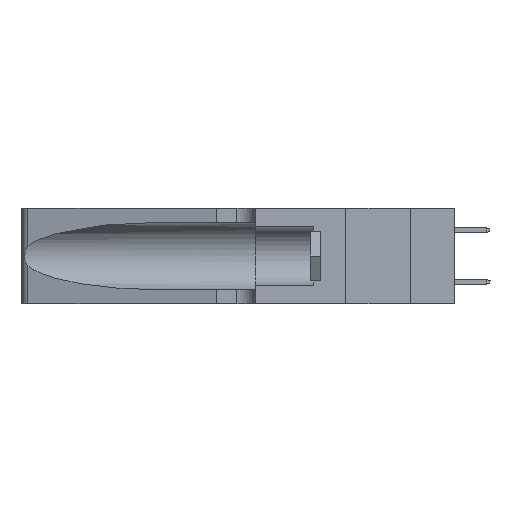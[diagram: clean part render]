
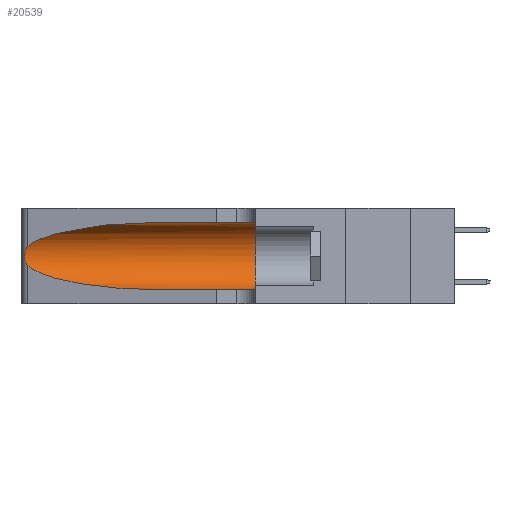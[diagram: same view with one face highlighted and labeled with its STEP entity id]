
A CAD part, left-side view. The second image highlights one B-rep face of the part: STEP entity #20539.
In plain terms, the highlighted cylindrical face has radius 3.308 mm (diameter 6.617 mm), a partial arc.
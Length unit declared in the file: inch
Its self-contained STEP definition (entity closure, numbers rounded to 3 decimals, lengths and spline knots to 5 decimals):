
#292 = CARTESIAN_POINT ( 'NONE',  ( 0.26075, 1.23896, 0.19203 ) ) ;
#440 = AXIS2_PLACEMENT_3D ( 'NONE', #18589, #21088, #26105 ) ;
#1150 = DIRECTION ( 'NONE',  ( 0., 0., -1. ) ) ;
#2036 = CARTESIAN_POINT ( 'NONE',  ( 0.1305, 0.72297, 0.05475 ) ) ;
#2188 = CARTESIAN_POINT ( 'NONE',  ( 0.1305, 1.61858, 0.31525 ) ) ;
#2453 = CARTESIAN_POINT ( 'NONE',  ( 0.25487, 1.22718, 0.22369 ) ) ;
#2631 = CARTESIAN_POINT ( 'NONE',  ( 0.25555, 1.22993, 0.14849 ) ) ;
#2704 = CARTESIAN_POINT ( 'NONE',  ( 0.1305, 0.35, 0.31525 ) ) ;
#2772 = CARTESIAN_POINT ( 'NONE',  ( 0.25787, 1.23484, 0.2124 ) ) ;
#3250 = VERTEX_POINT ( 'NONE', #12655 ) ;
#3545 = EDGE_CURVE ( 'NONE', #10088, #3250, #20313, .T. ) ;
#3621 = ORIENTED_EDGE ( 'NONE', *, *, #28173, .T. ) ;
#3912 = ORIENTED_EDGE ( 'NONE', *, *, #11905, .T. ) ;
#4317 = CARTESIAN_POINT ( 'NONE',  ( 0.25487, 1.22718, 0.22369 ) ) ;
#4674 = CARTESIAN_POINT ( 'NONE',  ( 0.2373, 1.15595, 0.08982 ) ) ;
#5006 = CARTESIAN_POINT ( 'NONE',  ( 0.25487, 1.22718, 0.14631 ) ) ;
#5049 = LINE ( 'NONE', #23955, #10799 ) ;
#5789 = FACE_OUTER_BOUND ( 'NONE', #12673, .T. ) ;
#5851 =( BOUNDED_CURVE ( )  B_SPLINE_CURVE ( 3, ( #9763, #19253, #19100, #2453 ),
 .UNSPECIFIED., .F., .F. ) 
 B_SPLINE_CURVE_WITH_KNOTS ( ( 4, 4 ),
 ( 1.5708, 2.84003 ),
 .UNSPECIFIED. ) 
 CURVE ( )  GEOMETRIC_REPRESENTATION_ITEM ( )  RATIONAL_B_SPLINE_CURVE ( ( 1., 0.87, 0.87, 1. ) ) 
 REPRESENTATION_ITEM ( '' )  );
#8058 =( BOUNDED_CURVE ( )  B_SPLINE_CURVE ( 3, ( #30767, #4674, #9676, #19167 ),
 .UNSPECIFIED., .F., .F. ) 
 B_SPLINE_CURVE_WITH_KNOTS ( ( 4, 4 ),
 ( 3.44316, 4.71239 ),
 .UNSPECIFIED. ) 
 CURVE ( )  GEOMETRIC_REPRESENTATION_ITEM ( )  RATIONAL_B_SPLINE_CURVE ( ( 1., 0.87, 0.87, 1. ) ) 
 REPRESENTATION_ITEM ( '' )  );
#8305 = DIRECTION ( 'NONE',  ( 0., -1., 0. ) ) ;
#8444 = CARTESIAN_POINT ( 'NONE',  ( 0.25487, 1.22718, 0.22369 ) ) ;
#9632 = CARTESIAN_POINT ( 'NONE',  ( 0.26018, 1.23835, 0.19895 ) ) ;
#9676 = CARTESIAN_POINT ( 'NONE',  ( 0.18966, 0.96281, 0.05475 ) ) ;
#9763 = CARTESIAN_POINT ( 'NONE',  ( 0.1305, 0.72297, 0.31525 ) ) ;
#9938 = CARTESIAN_POINT ( 'NONE',  ( 0.25789, 1.23486, 0.15765 ) ) ;
#10088 = VERTEX_POINT ( 'NONE', #2704 ) ;
#10491 = CARTESIAN_POINT ( 'NONE',  ( 0.1305, 1.61858, 0.185 ) ) ;
#10799 = VECTOR ( 'NONE', #21581, 39.37008 ) ;
#10897 = ORIENTED_EDGE ( 'NONE', *, *, #3545, .F. ) ;
#11684 = ORIENTED_EDGE ( 'NONE', *, *, #16822, .T. ) ;
#11905 = EDGE_CURVE ( 'NONE', #28494, #29939, #8058, .T. ) ;
#12655 = CARTESIAN_POINT ( 'NONE',  ( 0.1305, 0.35, 0.05475 ) ) ;
#12673 = EDGE_LOOP ( 'NONE', ( #20501, #11684, #3912, #3621, #10897, #16724 ) ) ;
#13839 = CARTESIAN_POINT ( 'NONE',  ( 0.25555, 1.22994, 0.2215 ) ) ;
#14465 = CARTESIAN_POINT ( 'NONE',  ( 0.25856, 1.23593, 0.16098 ) ) ;
#14610 = CARTESIAN_POINT ( 'NONE',  ( 0.25639, 1.23186, 0.15144 ) ) ;
#15311 = CYLINDRICAL_SURFACE ( 'NONE', #25930, 0.13025 ) ;
#15328 = CARTESIAN_POINT ( 'NONE',  ( 0.25639, 1.23184, 0.21858 ) ) ;
#16203 = VERTEX_POINT ( 'NONE', #8444 ) ;
#16653 = CARTESIAN_POINT ( 'NONE',  ( 0.26075, 1.23896, 0.178 ) ) ;
#16724 = ORIENTED_EDGE ( 'NONE', *, *, #19316, .F. ) ;
#16822 = EDGE_CURVE ( 'NONE', #16203, #28494, #28674, .T. ) ;
#18564 = EDGE_CURVE ( 'NONE', #23115, #16203, #5851, .T. ) ;
#18589 = CARTESIAN_POINT ( 'NONE',  ( 0.1305, 0.35, 0.185 ) ) ;
#19100 = CARTESIAN_POINT ( 'NONE',  ( 0.2373, 1.15595, 0.28018 ) ) ;
#19123 = CARTESIAN_POINT ( 'NONE',  ( 0.26017, 1.23833, 0.17102 ) ) ;
#19167 = CARTESIAN_POINT ( 'NONE',  ( 0.1305, 0.72297, 0.05475 ) ) ;
#19253 = CARTESIAN_POINT ( 'NONE',  ( 0.18966, 0.96281, 0.31525 ) ) ;
#19316 = EDGE_CURVE ( 'NONE', #23115, #10088, #25751, .T. ) ;
#20313 = CIRCLE ( 'NONE', #440, 0.13025 ) ;
#20501 = ORIENTED_EDGE ( 'NONE', *, *, #18564, .T. ) ;
#20539 = ADVANCED_FACE ( 'NONE', ( #5789 ), #15311, .F. ) ;
#21088 = DIRECTION ( 'NONE',  ( 0., 1., 0. ) ) ;
#21482 = CARTESIAN_POINT ( 'NONE',  ( 0.25487, 1.22718, 0.14631 ) ) ;
#21581 = DIRECTION ( 'NONE',  ( 0., -1., 0. ) ) ;
#21623 = CARTESIAN_POINT ( 'NONE',  ( 0.25854, 1.2359, 0.20912 ) ) ;
#23115 = VERTEX_POINT ( 'NONE', #29186 ) ;
#23368 = VECTOR ( 'NONE', #30419, 39.37008 ) ;
#23955 = CARTESIAN_POINT ( 'NONE',  ( 0.1305, 1.61858, 0.05475 ) ) ;
#25751 = LINE ( 'NONE', #2188, #23368 ) ;
#25930 = AXIS2_PLACEMENT_3D ( 'NONE', #10491, #8305, #1150 ) ;
#26105 = DIRECTION ( 'NONE',  ( 0., 0., 1. ) ) ;
#28173 = EDGE_CURVE ( 'NONE', #29939, #3250, #5049, .T. ) ;
#28494 = VERTEX_POINT ( 'NONE', #5006 ) ;
#28674 = B_SPLINE_CURVE_WITH_KNOTS ( 'NONE', 3,
 ( #4317, #13839, #15328, #2772, #21623, #9632, #292, #16653, #19123, #14465, #9938, #14610, #2631, #21482 ),
 .UNSPECIFIED., .F., .F.,
 ( 4, 2, 2, 2, 2, 2, 4 ),
 ( 0., 0.00027, 0.00053, 0.00107, 0.0016, 0.00187, 0.00214 ),
 .UNSPECIFIED. ) ;
#29186 = CARTESIAN_POINT ( 'NONE',  ( 0.1305, 0.72297, 0.31525 ) ) ;
#29939 = VERTEX_POINT ( 'NONE', #2036 ) ;
#30419 = DIRECTION ( 'NONE',  ( 0., -1., 0. ) ) ;
#30767 = CARTESIAN_POINT ( 'NONE',  ( 0.25487, 1.22718, 0.14631 ) ) ;
